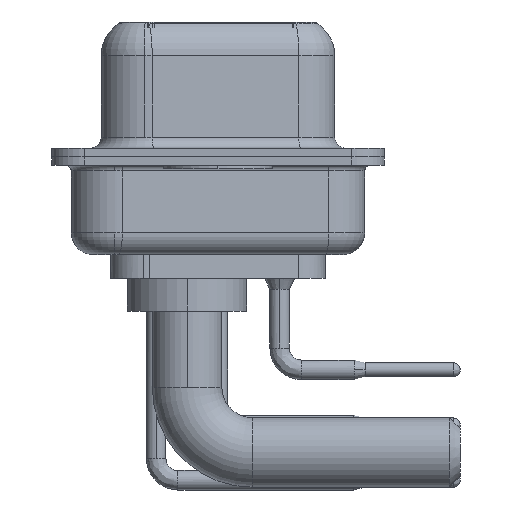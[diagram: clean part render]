
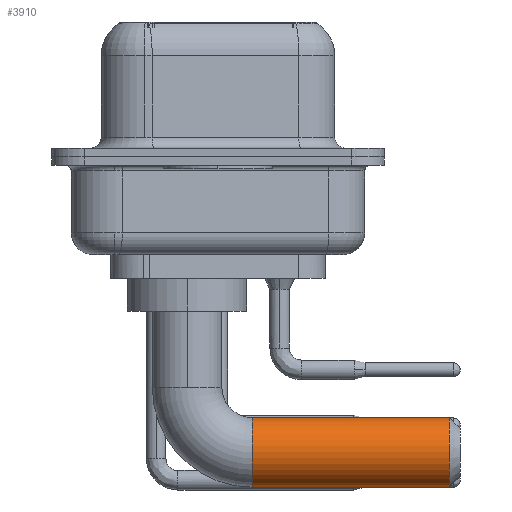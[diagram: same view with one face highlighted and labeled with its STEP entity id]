
A CAD part, left-side view. The second image highlights one B-rep face of the part: STEP entity #3910.
In plain terms, the highlighted cylindrical face has radius 1.6 mm (diameter 3.2 mm), a partial arc.
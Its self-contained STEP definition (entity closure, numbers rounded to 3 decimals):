
#105 = EDGE_LOOP ( 'NONE', ( #7476, #28827, #25386, #19750 ) ) ;
#1157 = VECTOR ( 'NONE', #22077, 1000. ) ;
#3682 = VERTEX_POINT ( 'NONE', #9304 ) ;
#3899 = DIRECTION ( 'NONE',  ( 0., 0., -1. ) ) ;
#3910 = ADVANCED_FACE ( 'NONE', ( #8300 ), #21332, .T. ) ;
#4168 = CARTESIAN_POINT ( 'NONE',  ( 0., -3., -4.9 ) ) ;
#5352 = VERTEX_POINT ( 'NONE', #11203 ) ;
#5373 = DIRECTION ( 'NONE',  ( -1., 0., 0. ) ) ;
#7476 = ORIENTED_EDGE ( 'NONE', *, *, #27728, .F. ) ;
#7556 = DIRECTION ( 'NONE',  ( 0., 1., 0. ) ) ;
#8300 = FACE_OUTER_BOUND ( 'NONE', #105, .T. ) ;
#9022 = AXIS2_PLACEMENT_3D ( 'NONE', #22236, #7556, #22889 ) ;
#9304 = CARTESIAN_POINT ( 'NONE',  ( 0., -3., -4.9 ) ) ;
#10850 = LINE ( 'NONE', #16068, #12228 ) ;
#11203 = CARTESIAN_POINT ( 'NONE',  ( 0., -12.07, -4.9 ) ) ;
#12228 = VECTOR ( 'NONE', #26009, 1000. ) ;
#15801 = DIRECTION ( 'NONE',  ( 0., -1., 0. ) ) ;
#16068 = CARTESIAN_POINT ( 'NONE',  ( 0., -3., -8.1 ) ) ;
#17089 = VERTEX_POINT ( 'NONE', #23190 ) ;
#19406 = EDGE_CURVE ( 'NONE', #17089, #28936, #10850, .T. ) ;
#19750 = ORIENTED_EDGE ( 'NONE', *, *, #28006, .T. ) ;
#20499 = AXIS2_PLACEMENT_3D ( 'NONE', #25595, #30464, #5373 ) ;
#21332 = CYLINDRICAL_SURFACE ( 'NONE', #28820, 1.6 ) ;
#22077 = DIRECTION ( 'NONE',  ( 0., -1., 0. ) ) ;
#22236 = CARTESIAN_POINT ( 'NONE',  ( 0., -12.07, -6.5 ) ) ;
#22889 = DIRECTION ( 'NONE',  ( 0., 0., -1. ) ) ;
#23190 = CARTESIAN_POINT ( 'NONE',  ( 0., -3., -8.1 ) ) ;
#24626 = CIRCLE ( 'NONE', #9022, 1.6 ) ;
#25386 = ORIENTED_EDGE ( 'NONE', *, *, #19406, .T. ) ;
#25595 = CARTESIAN_POINT ( 'NONE',  ( 0., -3., -6.5 ) ) ;
#26009 = DIRECTION ( 'NONE',  ( 0., -1., 0. ) ) ;
#26661 = LINE ( 'NONE', #4168, #1157 ) ;
#27728 = EDGE_CURVE ( 'NONE', #3682, #5352, #26661, .T. ) ;
#28006 = EDGE_CURVE ( 'NONE', #28936, #5352, #24626, .T. ) ;
#28677 = CARTESIAN_POINT ( 'NONE',  ( 0., -3., -6.5 ) ) ;
#28820 = AXIS2_PLACEMENT_3D ( 'NONE', #28677, #15801, #3899 ) ;
#28827 = ORIENTED_EDGE ( 'NONE', *, *, #31589, .T. ) ;
#28936 = VERTEX_POINT ( 'NONE', #28949 ) ;
#28949 = CARTESIAN_POINT ( 'NONE',  ( 0., -12.07, -8.1 ) ) ;
#30464 = DIRECTION ( 'NONE',  ( 0., -1., 0. ) ) ;
#31589 = EDGE_CURVE ( 'NONE', #3682, #17089, #31931, .T. ) ;
#31931 = CIRCLE ( 'NONE', #20499, 1.6 ) ;
